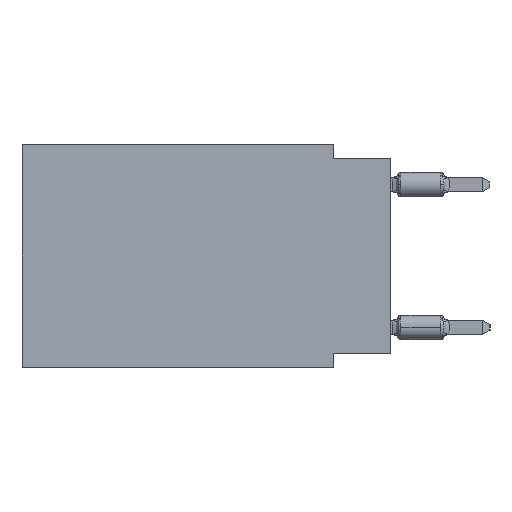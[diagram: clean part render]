
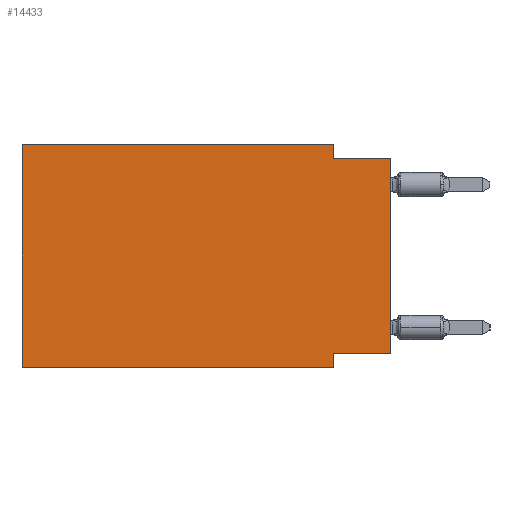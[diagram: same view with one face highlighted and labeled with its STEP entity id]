
A CAD part, left-side view. The second image highlights one B-rep face of the part: STEP entity #14433.
In plain terms, the highlighted planar face has unit normal (-1, 0, 0).
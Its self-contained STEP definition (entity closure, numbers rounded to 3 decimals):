
#237 = CARTESIAN_POINT ( 'NONE',  ( 0., 2.54, 0. ) ) ;
#690 = EDGE_CURVE ( 'NONE', #25734, #15788, #26856, .T. ) ;
#734 = CARTESIAN_POINT ( 'NONE',  ( 0., 2.54, -9.906 ) ) ;
#1434 = EDGE_CURVE ( 'NONE', #7336, #20703, #11770, .T. ) ;
#1576 = VERTEX_POINT ( 'NONE', #5973 ) ;
#3594 = ORIENTED_EDGE ( 'NONE', *, *, #12621, .F. ) ;
#3824 = DIRECTION ( 'NONE',  ( 1., 0., 0. ) ) ;
#3836 = EDGE_CURVE ( 'NONE', #26605, #7336, #23592, .T. ) ;
#3958 = ORIENTED_EDGE ( 'NONE', *, *, #690, .F. ) ;
#4418 = CARTESIAN_POINT ( 'NONE',  ( 0., 16.383, 0. ) ) ;
#4615 = CARTESIAN_POINT ( 'NONE',  ( 0., 16.383, -9.906 ) ) ;
#5973 = CARTESIAN_POINT ( 'NONE',  ( 0., 0., -0.635 ) ) ;
#5978 = PLANE ( 'NONE',  #26332 ) ;
#6217 = DIRECTION ( 'NONE',  ( 0., -1., 0. ) ) ;
#6770 = ORIENTED_EDGE ( 'NONE', *, *, #3836, .F. ) ;
#6989 = DIRECTION ( 'NONE',  ( 0., 0., 1. ) ) ;
#7336 = VERTEX_POINT ( 'NONE', #237 ) ;
#7621 = ORIENTED_EDGE ( 'NONE', *, *, #25405, .F. ) ;
#7972 = CARTESIAN_POINT ( 'NONE',  ( 0., 2.54, 0. ) ) ;
#8619 = VECTOR ( 'NONE', #13644, 1000. ) ;
#8808 = VECTOR ( 'NONE', #18510, 1000. ) ;
#8910 = DIRECTION ( 'NONE',  ( 0., -1., 0. ) ) ;
#9151 = VECTOR ( 'NONE', #28249, 1000. ) ;
#9425 = ORIENTED_EDGE ( 'NONE', *, *, #19651, .T. ) ;
#10292 = CARTESIAN_POINT ( 'NONE',  ( 0., 16.383, 0. ) ) ;
#10859 = ORIENTED_EDGE ( 'NONE', *, *, #1434, .F. ) ;
#11163 = LINE ( 'NONE', #4418, #9151 ) ;
#11627 = CARTESIAN_POINT ( 'NONE',  ( 0., 0., -0.635 ) ) ;
#11770 = LINE ( 'NONE', #7972, #22881 ) ;
#12454 = CARTESIAN_POINT ( 'NONE',  ( 0., 16.383, -9.906 ) ) ;
#12621 = EDGE_CURVE ( 'NONE', #20703, #1576, #24985, .T. ) ;
#13327 = VECTOR ( 'NONE', #6989, 1000. ) ;
#13339 = VECTOR ( 'NONE', #19163, 1000. ) ;
#13644 = DIRECTION ( 'NONE',  ( 0., 0., -1. ) ) ;
#13744 = CARTESIAN_POINT ( 'NONE',  ( 0., 0., -9.271 ) ) ;
#14388 = VERTEX_POINT ( 'NONE', #27795 ) ;
#14390 = CARTESIAN_POINT ( 'NONE',  ( 0., 2.54, -0.635 ) ) ;
#14433 = ADVANCED_FACE ( 'NONE', ( #23923 ), #5978, .F. ) ;
#14894 = EDGE_CURVE ( 'NONE', #14388, #1576, #18331, .T. ) ;
#15743 = ORIENTED_EDGE ( 'NONE', *, *, #27001, .F. ) ;
#15788 = VERTEX_POINT ( 'NONE', #24578 ) ;
#18331 = LINE ( 'NONE', #26663, #13327 ) ;
#18335 = VECTOR ( 'NONE', #6217, 1000. ) ;
#18510 = DIRECTION ( 'NONE',  ( 0., -1., 0. ) ) ;
#19163 = DIRECTION ( 'NONE',  ( 0., 1., 0. ) ) ;
#19651 = EDGE_CURVE ( 'NONE', #26682, #15788, #19689, .T. ) ;
#19689 = LINE ( 'NONE', #4615, #21473 ) ;
#19976 = ORIENTED_EDGE ( 'NONE', *, *, #14894, .T. ) ;
#20703 = VERTEX_POINT ( 'NONE', #14390 ) ;
#20919 = CARTESIAN_POINT ( 'NONE',  ( 0., 2.54, -9.271 ) ) ;
#21473 = VECTOR ( 'NONE', #8910, 1000. ) ;
#22346 = LINE ( 'NONE', #13744, #13339 ) ;
#22881 = VECTOR ( 'NONE', #26846, 1000. ) ;
#22974 = EDGE_LOOP ( 'NONE', ( #19976, #3594, #10859, #6770, #7621, #9425, #3958, #15743 ) ) ;
#23485 = CARTESIAN_POINT ( 'NONE',  ( 0., 16.383, 0. ) ) ;
#23592 = LINE ( 'NONE', #25893, #18335 ) ;
#23777 = DIRECTION ( 'NONE',  ( 0., 0., -1. ) ) ;
#23923 = FACE_OUTER_BOUND ( 'NONE', #22974, .T. ) ;
#24578 = CARTESIAN_POINT ( 'NONE',  ( 0., 2.54, -9.906 ) ) ;
#24985 = LINE ( 'NONE', #11627, #8808 ) ;
#25405 = EDGE_CURVE ( 'NONE', #26682, #26605, #11163, .T. ) ;
#25734 = VERTEX_POINT ( 'NONE', #20919 ) ;
#25893 = CARTESIAN_POINT ( 'NONE',  ( 0., 16.383, 0. ) ) ;
#26332 = AXIS2_PLACEMENT_3D ( 'NONE', #23485, #3824, #23777 ) ;
#26605 = VERTEX_POINT ( 'NONE', #10292 ) ;
#26663 = CARTESIAN_POINT ( 'NONE',  ( 0., 0., 0. ) ) ;
#26682 = VERTEX_POINT ( 'NONE', #12454 ) ;
#26846 = DIRECTION ( 'NONE',  ( 0., 0., -1. ) ) ;
#26856 = LINE ( 'NONE', #734, #8619 ) ;
#27001 = EDGE_CURVE ( 'NONE', #14388, #25734, #22346, .T. ) ;
#27795 = CARTESIAN_POINT ( 'NONE',  ( 0., 0., -9.271 ) ) ;
#28249 = DIRECTION ( 'NONE',  ( 0., 0., 1. ) ) ;
